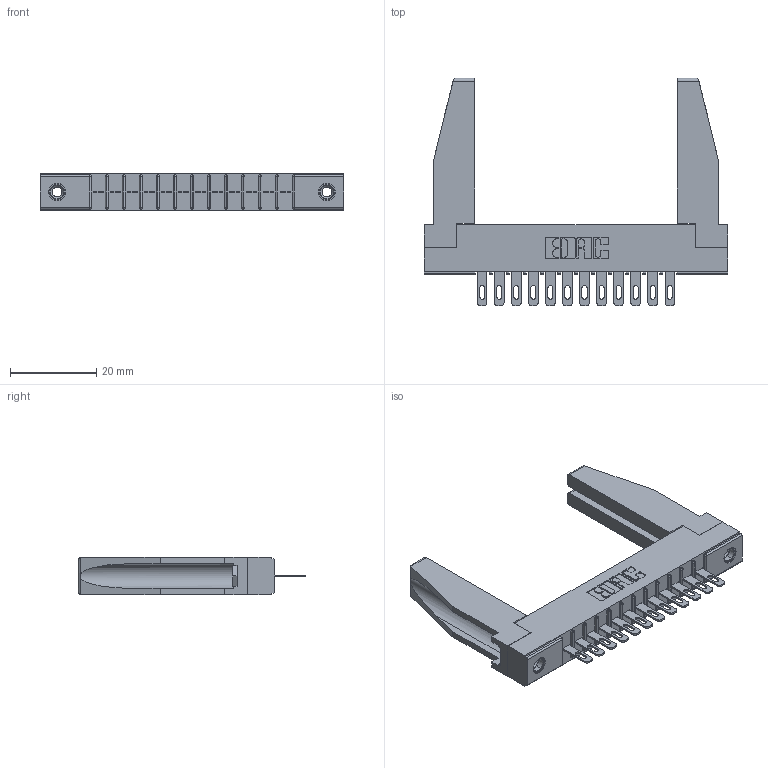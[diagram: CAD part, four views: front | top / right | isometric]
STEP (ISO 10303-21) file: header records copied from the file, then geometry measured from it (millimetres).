
FILE_DESCRIPTION (( 'STEP AP203' ), '1' );
FILE_NAME ('306-012-500-178.STEP', '2019-09-11T19:31:52', ( '' ), ( '' ), 'SwSTEP 2.0', 'SolidWorks 2016', '' );
FILE_SCHEMA (( 'CONFIG_CONTROL_DESIGN' ));
Length unit declared in the file: inch
Products named in the file (5): 306 Part_.156 Dia; 306-012-500-178; 306-290-001_100; 307-220-078; 345-250-001_345-250-001-102
Assembly tree (17 placements, depth 2):
  306-012-500-178
    306 Part_.156 Dia
    306-290-001_100  x12
    345-250-001_345-250-001-102  x2
    307-220-078  x2
Bounding box: 70.56 x 52.91 x 8.71 mm (x, y, z)
Volume: 8809.7 mm3; surface area: 10835.2 mm2
Topology: 17 solids, 17 shells, 1158 faces, 3226 edges, 2076 vertices
Faces by surface type: plane 752, cylinder 342, sphere 48, cone 12, torus 4
Entity records: 17680 total; most frequent: CARTESIAN_POINT 2965, ORIENTED_EDGE 2894, DIRECTION 2879, EDGE_CURVE 1447, LINE 1115, VECTOR 1115, VERTEX_POINT 926, AXIS2_PLACEMENT_3D 882
